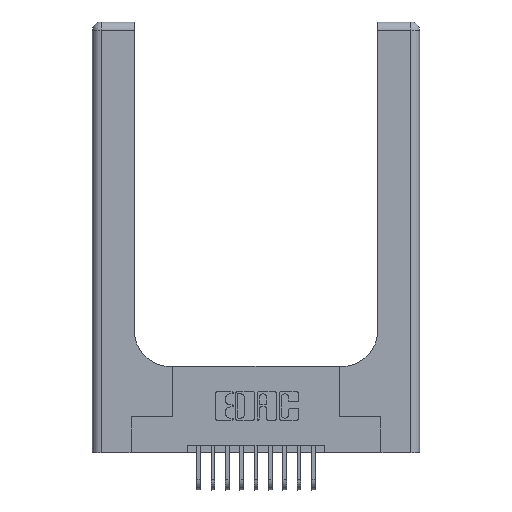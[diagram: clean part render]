
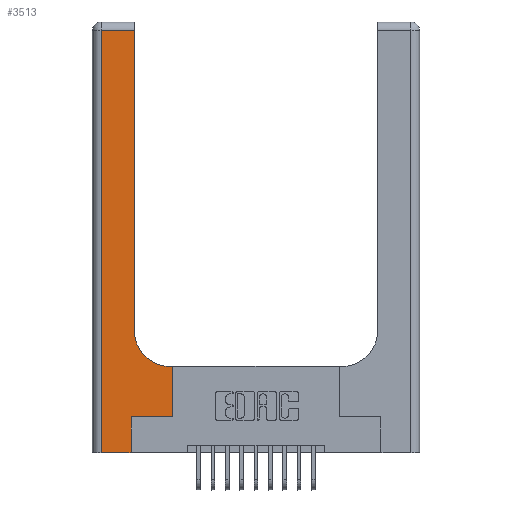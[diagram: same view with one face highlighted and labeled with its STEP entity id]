
A CAD part, top view. The second image highlights one B-rep face of the part: STEP entity #3513.
In plain terms, the highlighted planar face has unit normal (0, 0, 1).
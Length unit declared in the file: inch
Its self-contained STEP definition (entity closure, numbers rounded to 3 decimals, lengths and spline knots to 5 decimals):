
#34 = VERTEX_POINT ( 'NONE', #8770 ) ;
#52 = DIRECTION ( 'NONE',  ( 0., 1., 0. ) ) ;
#298 = VERTEX_POINT ( 'NONE', #12376 ) ;
#484 = CARTESIAN_POINT ( 'NONE',  ( 0.2915, 0.6, 0.37 ) ) ;
#506 = EDGE_CURVE ( 'NONE', #13290, #34, #17508, .T. ) ;
#869 = AXIS2_PLACEMENT_3D ( 'NONE', #13263, #4928, #14665 ) ;
#1560 = LINE ( 'NONE', #11480, #8815 ) ;
#1600 = ORIENTED_EDGE ( 'NONE', *, *, #9236, .T. ) ;
#1995 = DIRECTION ( 'NONE',  ( -1., 0., 0. ) ) ;
#2023 = ORIENTED_EDGE ( 'NONE', *, *, #8781, .T. ) ;
#3268 = CARTESIAN_POINT ( 'NONE',  ( 0.06, 3., 0.37 ) ) ;
#3407 = CARTESIAN_POINT ( 'NONE',  ( 0.5585, 0.25, 0.37 ) ) ;
#3513 = ADVANCED_FACE ( 'NONE', ( #14823 ), #9155, .F. ) ;
#3989 = LINE ( 'NONE', #484, #17985 ) ;
#4412 = ORIENTED_EDGE ( 'NONE', *, *, #12084, .T. ) ;
#4928 = DIRECTION ( 'NONE',  ( 0., 0., -1. ) ) ;
#5285 = ORIENTED_EDGE ( 'NONE', *, *, #14621, .T. ) ;
#5406 = CARTESIAN_POINT ( 'NONE',  ( 0.2915, 3., 0.37 ) ) ;
#5513 = DIRECTION ( 'NONE',  ( 0., -1., 0. ) ) ;
#5845 = CARTESIAN_POINT ( 'NONE',  ( 0.5585, 0.25, 0.37 ) ) ;
#6006 = DIRECTION ( 'NONE',  ( 1., 0., 0. ) ) ;
#6327 = ORIENTED_EDGE ( 'NONE', *, *, #506, .T. ) ;
#6424 = EDGE_CURVE ( 'NONE', #34, #14097, #9148, .T. ) ;
#6471 = ORIENTED_EDGE ( 'NONE', *, *, #6424, .T. ) ;
#6873 = DIRECTION ( 'NONE',  ( 0., 1., 0. ) ) ;
#7018 = VERTEX_POINT ( 'NONE', #14226 ) ;
#7054 = CARTESIAN_POINT ( 'NONE',  ( 0.2915, 0.85, 0.37 ) ) ;
#7609 = VERTEX_POINT ( 'NONE', #5845 ) ;
#8098 = ORIENTED_EDGE ( 'NONE', *, *, #12075, .T. ) ;
#8168 = CARTESIAN_POINT ( 'NONE',  ( 0.269, 0.25, 0.37 ) ) ;
#8387 = CARTESIAN_POINT ( 'NONE',  ( 0.5415, 0.85, 0.37 ) ) ;
#8770 = CARTESIAN_POINT ( 'NONE',  ( 0.06, 0., 0.37 ) ) ;
#8781 = EDGE_CURVE ( 'NONE', #10814, #13290, #9264, .T. ) ;
#8815 = VECTOR ( 'NONE', #52, 39.37008 ) ;
#8826 = ORIENTED_EDGE ( 'NONE', *, *, #15004, .T. ) ;
#8843 = CARTESIAN_POINT ( 'NONE',  ( 0.269, 0.25, 0.37 ) ) ;
#9046 = LINE ( 'NONE', #5406, #15948 ) ;
#9065 = VERTEX_POINT ( 'NONE', #7054 ) ;
#9148 = LINE ( 'NONE', #14369, #12332 ) ;
#9155 = PLANE ( 'NONE',  #869 ) ;
#9236 = EDGE_CURVE ( 'NONE', #14097, #14959, #1560, .T. ) ;
#9264 = LINE ( 'NONE', #10325, #12014 ) ;
#9333 = ORIENTED_EDGE ( 'NONE', *, *, #16447, .T. ) ;
#9762 = DIRECTION ( 'NONE',  ( 1., 0., 0. ) ) ;
#10325 = CARTESIAN_POINT ( 'NONE',  ( 0., 2.94, 0.37 ) ) ;
#10540 = VECTOR ( 'NONE', #6006, 39.37008 ) ;
#10814 = VERTEX_POINT ( 'NONE', #14142 ) ;
#11480 = CARTESIAN_POINT ( 'NONE',  ( 0.269, 0., 0.37 ) ) ;
#12014 = VECTOR ( 'NONE', #17234, 39.37008 ) ;
#12075 = EDGE_CURVE ( 'NONE', #7609, #7018, #15172, .T. ) ;
#12084 = EDGE_CURVE ( 'NONE', #7018, #298, #3989, .T. ) ;
#12332 = VECTOR ( 'NONE', #15787, 39.37008 ) ;
#12376 = CARTESIAN_POINT ( 'NONE',  ( 0.5415, 0.6, 0.37 ) ) ;
#12552 = CIRCLE ( 'NONE', #15836, 0.25 ) ;
#13263 = CARTESIAN_POINT ( 'NONE',  ( 0., 3., 0.37 ) ) ;
#13290 = VERTEX_POINT ( 'NONE', #16068 ) ;
#13638 = CARTESIAN_POINT ( 'NONE',  ( 0.269, 0., 0.37 ) ) ;
#14097 = VERTEX_POINT ( 'NONE', #13638 ) ;
#14142 = CARTESIAN_POINT ( 'NONE',  ( 0.2915, 2.94, 0.37 ) ) ;
#14226 = CARTESIAN_POINT ( 'NONE',  ( 0.5585, 0.6, 0.37 ) ) ;
#14369 = CARTESIAN_POINT ( 'NONE',  ( 0., 0., 0.37 ) ) ;
#14621 = EDGE_CURVE ( 'NONE', #14959, #7609, #18318, .T. ) ;
#14634 = DIRECTION ( 'NONE',  ( 0., 1., 0. ) ) ;
#14665 = DIRECTION ( 'NONE',  ( -1., 0., 0. ) ) ;
#14679 = VECTOR ( 'NONE', #5513, 39.37008 ) ;
#14720 = VECTOR ( 'NONE', #14634, 39.37008 ) ;
#14823 = FACE_OUTER_BOUND ( 'NONE', #15957, .T. ) ;
#14959 = VERTEX_POINT ( 'NONE', #8168 ) ;
#15004 = EDGE_CURVE ( 'NONE', #9065, #10814, #9046, .T. ) ;
#15172 = LINE ( 'NONE', #3407, #14720 ) ;
#15787 = DIRECTION ( 'NONE',  ( 1., 0., 0. ) ) ;
#15836 = AXIS2_PLACEMENT_3D ( 'NONE', #8387, #18042, #9762 ) ;
#15948 = VECTOR ( 'NONE', #6873, 39.37008 ) ;
#15957 = EDGE_LOOP ( 'NONE', ( #8826, #2023, #6327, #6471, #1600, #5285, #8098, #4412, #9333 ) ) ;
#16068 = CARTESIAN_POINT ( 'NONE',  ( 0.06, 2.94, 0.37 ) ) ;
#16447 = EDGE_CURVE ( 'NONE', #298, #9065, #12552, .T. ) ;
#17234 = DIRECTION ( 'NONE',  ( -1., 0., 0. ) ) ;
#17508 = LINE ( 'NONE', #3268, #14679 ) ;
#17985 = VECTOR ( 'NONE', #1995, 39.37008 ) ;
#18042 = DIRECTION ( 'NONE',  ( 0., 0., -1. ) ) ;
#18318 = LINE ( 'NONE', #8843, #10540 ) ;
